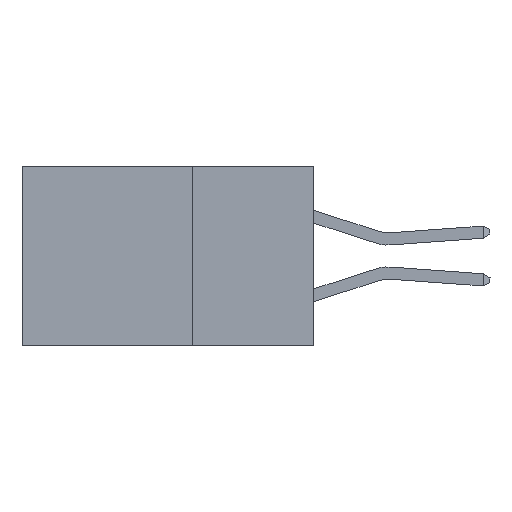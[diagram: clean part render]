
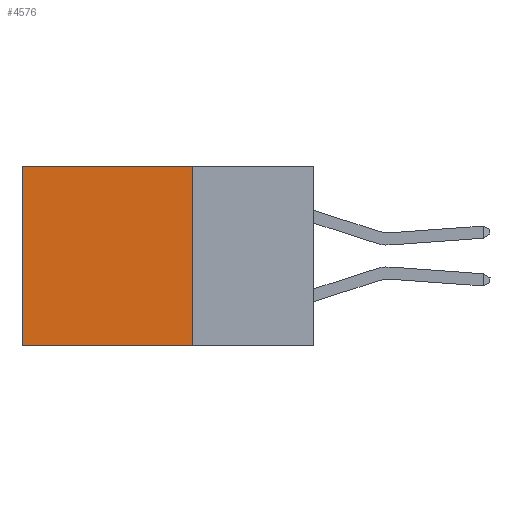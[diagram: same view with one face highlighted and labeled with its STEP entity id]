
A CAD part, left-side view. The second image highlights one B-rep face of the part: STEP entity #4576.
In plain terms, the highlighted planar face has unit normal (-1, 0, 0).
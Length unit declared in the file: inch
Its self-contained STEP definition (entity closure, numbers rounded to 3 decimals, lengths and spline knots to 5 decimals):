
#1258 = VECTOR ( 'NONE', #14725, 39.37008 ) ;
#2324 = LINE ( 'NONE', #22367, #6139 ) ;
#2690 = DIRECTION ( 'NONE',  ( 0., 1., 0. ) ) ;
#3141 = EDGE_CURVE ( 'NONE', #22058, #22370, #7609, .T. ) ;
#4576 = ADVANCED_FACE ( 'NONE', ( #4735 ), #10761, .F. ) ;
#4735 = FACE_OUTER_BOUND ( 'NONE', #16228, .T. ) ;
#5872 = DIRECTION ( 'NONE',  ( 1., 0., 0. ) ) ;
#6139 = VECTOR ( 'NONE', #6346, 39.37008 ) ;
#6346 = DIRECTION ( 'NONE',  ( 0., 0., -1. ) ) ;
#7180 = ORIENTED_EDGE ( 'NONE', *, *, #22368, .F. ) ;
#7609 = LINE ( 'NONE', #21777, #15936 ) ;
#9844 = CARTESIAN_POINT ( 'NONE',  ( 0.2875, 0.25, 0. ) ) ;
#10020 = VECTOR ( 'NONE', #11916, 39.37008 ) ;
#10761 = PLANE ( 'NONE',  #16668 ) ;
#11701 = VERTEX_POINT ( 'NONE', #17407 ) ;
#11916 = DIRECTION ( 'NONE',  ( 0., 0., -1. ) ) ;
#13819 = CARTESIAN_POINT ( 'NONE',  ( 0.2875, 0.25, 0. ) ) ;
#14184 = VERTEX_POINT ( 'NONE', #20356 ) ;
#14725 = DIRECTION ( 'NONE',  ( 0., 1., 0. ) ) ;
#15029 = EDGE_CURVE ( 'NONE', #22370, #14184, #2324, .T. ) ;
#15936 = VECTOR ( 'NONE', #2690, 39.37008 ) ;
#16138 = LINE ( 'NONE', #13819, #10020 ) ;
#16216 = LINE ( 'NONE', #16875, #1258 ) ;
#16228 = EDGE_LOOP ( 'NONE', ( #21528, #7180, #17218, #20759 ) ) ;
#16668 = AXIS2_PLACEMENT_3D ( 'NONE', #9844, #5872, #26000 ) ;
#16875 = CARTESIAN_POINT ( 'NONE',  ( 0.2875, 0.25, -0.37 ) ) ;
#17218 = ORIENTED_EDGE ( 'NONE', *, *, #24046, .F. ) ;
#17407 = CARTESIAN_POINT ( 'NONE',  ( 0.2875, 0.25, -0.37 ) ) ;
#17705 = CARTESIAN_POINT ( 'NONE',  ( 0.2875, 0.25, 0. ) ) ;
#20356 = CARTESIAN_POINT ( 'NONE',  ( 0.2875, 0.6, -0.37 ) ) ;
#20759 = ORIENTED_EDGE ( 'NONE', *, *, #3141, .T. ) ;
#21528 = ORIENTED_EDGE ( 'NONE', *, *, #15029, .T. ) ;
#21777 = CARTESIAN_POINT ( 'NONE',  ( 0.2875, 0.25, 0. ) ) ;
#22058 = VERTEX_POINT ( 'NONE', #17705 ) ;
#22367 = CARTESIAN_POINT ( 'NONE',  ( 0.2875, 0.6, 0. ) ) ;
#22368 = EDGE_CURVE ( 'NONE', #11701, #14184, #16216, .T. ) ;
#22370 = VERTEX_POINT ( 'NONE', #22961 ) ;
#22961 = CARTESIAN_POINT ( 'NONE',  ( 0.2875, 0.6, 0. ) ) ;
#24046 = EDGE_CURVE ( 'NONE', #22058, #11701, #16138, .T. ) ;
#26000 = DIRECTION ( 'NONE',  ( 0., 0., -1. ) ) ;
